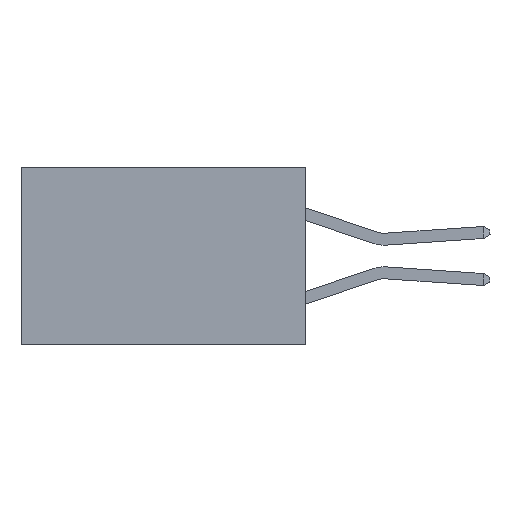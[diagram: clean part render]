
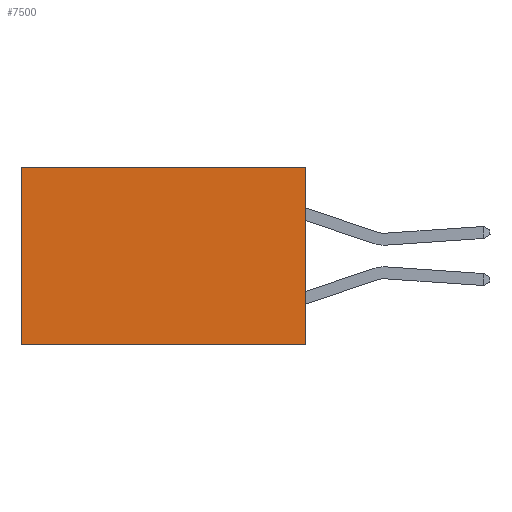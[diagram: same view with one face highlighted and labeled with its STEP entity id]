
A CAD part, left-side view. The second image highlights one B-rep face of the part: STEP entity #7500.
In plain terms, the highlighted planar face has unit normal (-1, 0, 0).
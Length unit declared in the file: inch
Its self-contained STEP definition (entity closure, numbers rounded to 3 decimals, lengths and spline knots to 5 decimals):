
#501 = FACE_OUTER_BOUND ( 'NONE', #979, .T. ) ;
#524 = DIRECTION ( 'NONE',  ( 0., 1., 0. ) ) ;
#979 = EDGE_LOOP ( 'NONE', ( #15261, #8568, #4834, #9531 ) ) ;
#1493 = VERTEX_POINT ( 'NONE', #9691 ) ;
#1608 = EDGE_CURVE ( 'NONE', #1493, #3249, #9294, .T. ) ;
#1745 = VECTOR ( 'NONE', #12585, 39.37008 ) ;
#1928 = EDGE_CURVE ( 'NONE', #12821, #4954, #11179, .T. ) ;
#2190 = DIRECTION ( 'NONE',  ( 0., 0., -1. ) ) ;
#3249 = VERTEX_POINT ( 'NONE', #13062 ) ;
#3829 = CARTESIAN_POINT ( 'NONE',  ( 0.277, 0.59, -0.37 ) ) ;
#4791 = EDGE_CURVE ( 'NONE', #3249, #4954, #18591, .T. ) ;
#4834 = ORIENTED_EDGE ( 'NONE', *, *, #17066, .F. ) ;
#4954 = VERTEX_POINT ( 'NONE', #3829 ) ;
#6522 = CARTESIAN_POINT ( 'NONE',  ( 0.277, 0., 0. ) ) ;
#6704 = VECTOR ( 'NONE', #13475, 39.37008 ) ;
#7254 = DIRECTION ( 'NONE',  ( 0., 0., -1. ) ) ;
#7500 = ADVANCED_FACE ( 'NONE', ( #501 ), #8594, .F. ) ;
#7614 = CARTESIAN_POINT ( 'NONE',  ( 0.277, 0.59, -0.37 ) ) ;
#8568 = ORIENTED_EDGE ( 'NONE', *, *, #1928, .F. ) ;
#8594 = PLANE ( 'NONE',  #11249 ) ;
#9294 = LINE ( 'NONE', #6522, #12856 ) ;
#9531 = ORIENTED_EDGE ( 'NONE', *, *, #1608, .T. ) ;
#9691 = CARTESIAN_POINT ( 'NONE',  ( 0.277, 0., 0. ) ) ;
#10126 = CARTESIAN_POINT ( 'NONE',  ( 0.277, 0., -0.37 ) ) ;
#11179 = LINE ( 'NONE', #13340, #1745 ) ;
#11249 = AXIS2_PLACEMENT_3D ( 'NONE', #10126, #11640, #2190 ) ;
#11640 = DIRECTION ( 'NONE',  ( 1., 0., 0. ) ) ;
#12585 = DIRECTION ( 'NONE',  ( 0., 1., 0. ) ) ;
#12821 = VERTEX_POINT ( 'NONE', #19349 ) ;
#12856 = VECTOR ( 'NONE', #524, 39.37008 ) ;
#13062 = CARTESIAN_POINT ( 'NONE',  ( 0.277, 0.59, 0. ) ) ;
#13340 = CARTESIAN_POINT ( 'NONE',  ( 0.277, 0., -0.37 ) ) ;
#13475 = DIRECTION ( 'NONE',  ( 0., 0., -1. ) ) ;
#14227 = VECTOR ( 'NONE', #7254, 39.37008 ) ;
#15013 = CARTESIAN_POINT ( 'NONE',  ( 0.277, 0., -0.37 ) ) ;
#15261 = ORIENTED_EDGE ( 'NONE', *, *, #4791, .T. ) ;
#17066 = EDGE_CURVE ( 'NONE', #1493, #12821, #18725, .T. ) ;
#18591 = LINE ( 'NONE', #7614, #14227 ) ;
#18725 = LINE ( 'NONE', #15013, #6704 ) ;
#19349 = CARTESIAN_POINT ( 'NONE',  ( 0.277, 0., -0.37 ) ) ;
